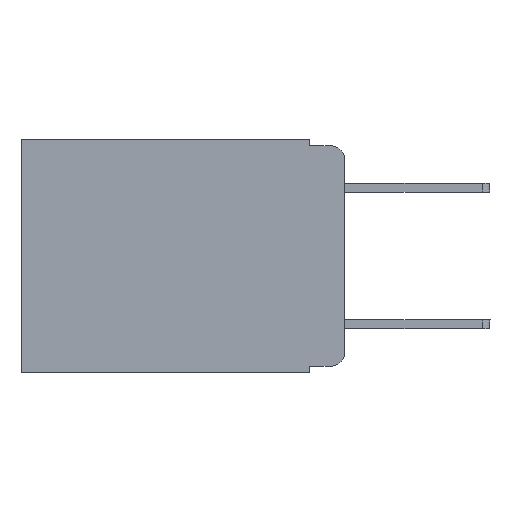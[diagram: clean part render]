
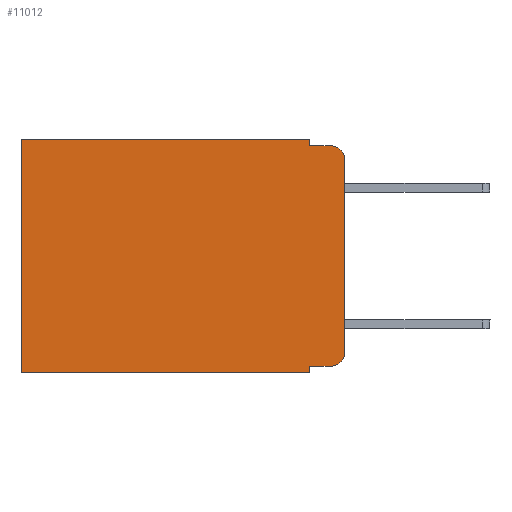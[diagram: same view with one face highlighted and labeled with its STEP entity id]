
A CAD part, left-side view. The second image highlights one B-rep face of the part: STEP entity #11012.
In plain terms, the highlighted planar face has unit normal (-1, 0, 0).
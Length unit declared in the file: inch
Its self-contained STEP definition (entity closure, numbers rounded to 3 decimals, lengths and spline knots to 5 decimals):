
#335 = VERTEX_POINT ( 'NONE', #15757 ) ;
#423 = VERTEX_POINT ( 'NONE', #14371 ) ;
#572 = VECTOR ( 'NONE', #6449, 39.37008 ) ;
#731 = EDGE_CURVE ( 'NONE', #1321, #17641, #1587, .T. ) ;
#1117 = EDGE_CURVE ( 'NONE', #423, #15335, #13544, .T. ) ;
#1249 = CARTESIAN_POINT ( 'NONE',  ( 0.298, 0.473, -0.343 ) ) ;
#1259 = VERTEX_POINT ( 'NONE', #11235 ) ;
#1321 = VERTEX_POINT ( 'NONE', #9311 ) ;
#1359 = LINE ( 'NONE', #6147, #572 ) ;
#1587 = LINE ( 'NONE', #19120, #15562 ) ;
#1827 = CARTESIAN_POINT ( 'NONE',  ( 0.298, 0.02, -0.03 ) ) ;
#2171 = CARTESIAN_POINT ( 'NONE',  ( 0.298, 0., -0.343 ) ) ;
#2373 = DIRECTION ( 'NONE',  ( 0., 1., 0. ) ) ;
#2409 = LINE ( 'NONE', #3792, #13209 ) ;
#2750 = CIRCLE ( 'NONE', #15293, 0.02 ) ;
#2806 = ORIENTED_EDGE ( 'NONE', *, *, #12698, .F. ) ;
#3792 = CARTESIAN_POINT ( 'NONE',  ( 0.298, 0.051, -0.01 ) ) ;
#3807 = CARTESIAN_POINT ( 'NONE',  ( 0.298, 0.02, -0.313 ) ) ;
#3870 = LINE ( 'NONE', #5986, #17325 ) ;
#3873 = EDGE_CURVE ( 'NONE', #10299, #15335, #6056, .T. ) ;
#4924 = VECTOR ( 'NONE', #15930, 39.37008 ) ;
#5332 = CARTESIAN_POINT ( 'NONE',  ( 0.298, 0.051, 0. ) ) ;
#5481 = DIRECTION ( 'NONE',  ( 1., 0., 0. ) ) ;
#5783 = ORIENTED_EDGE ( 'NONE', *, *, #17838, .T. ) ;
#5833 = VERTEX_POINT ( 'NONE', #1249 ) ;
#5986 = CARTESIAN_POINT ( 'NONE',  ( 0.298, 0.473, 0. ) ) ;
#6056 = LINE ( 'NONE', #10724, #9337 ) ;
#6147 = CARTESIAN_POINT ( 'NONE',  ( 0.298, 0.051, 0. ) ) ;
#6407 = EDGE_CURVE ( 'NONE', #7857, #423, #9598, .T. ) ;
#6449 = DIRECTION ( 'NONE',  ( 0., 0., -1. ) ) ;
#6607 = DIRECTION ( 'NONE',  ( 0., 0., -1. ) ) ;
#6977 = CARTESIAN_POINT ( 'NONE',  ( 0.298, 0., -0.313 ) ) ;
#7153 = DIRECTION ( 'NONE',  ( 0., 0., -1. ) ) ;
#7506 = VERTEX_POINT ( 'NONE', #8862 ) ;
#7857 = VERTEX_POINT ( 'NONE', #18734 ) ;
#8014 = CARTESIAN_POINT ( 'NONE',  ( 0.298, 0.051, -0.333 ) ) ;
#8066 = DIRECTION ( 'NONE',  ( 0., 1., 0. ) ) ;
#8364 = EDGE_CURVE ( 'NONE', #1321, #335, #12219, .T. ) ;
#8823 = ORIENTED_EDGE ( 'NONE', *, *, #8364, .F. ) ;
#8862 = CARTESIAN_POINT ( 'NONE',  ( 0.298, 0.051, -0.343 ) ) ;
#8982 = ORIENTED_EDGE ( 'NONE', *, *, #6407, .T. ) ;
#9311 = CARTESIAN_POINT ( 'NONE',  ( 0.298, 0.051, 0. ) ) ;
#9337 = VECTOR ( 'NONE', #13895, 39.37008 ) ;
#9350 = ORIENTED_EDGE ( 'NONE', *, *, #1117, .T. ) ;
#9598 = LINE ( 'NONE', #8014, #10572 ) ;
#10025 = FACE_OUTER_BOUND ( 'NONE', #13487, .T. ) ;
#10299 = VERTEX_POINT ( 'NONE', #19737 ) ;
#10348 = DIRECTION ( 'NONE',  ( 0., 0., -1. ) ) ;
#10572 = VECTOR ( 'NONE', #14577, 39.37008 ) ;
#10634 = ORIENTED_EDGE ( 'NONE', *, *, #3873, .F. ) ;
#10724 = CARTESIAN_POINT ( 'NONE',  ( 0.298, 0., 0. ) ) ;
#11012 = ADVANCED_FACE ( 'NONE', ( #10025 ), #16942, .F. ) ;
#11235 = CARTESIAN_POINT ( 'NONE',  ( 0.298, 0.02, -0.01 ) ) ;
#11397 = AXIS2_PLACEMENT_3D ( 'NONE', #13523, #5481, #10348 ) ;
#11866 = EDGE_CURVE ( 'NONE', #7857, #7506, #1359, .T. ) ;
#12219 = LINE ( 'NONE', #5332, #4924 ) ;
#12698 = EDGE_CURVE ( 'NONE', #7506, #5833, #16829, .T. ) ;
#13128 = VECTOR ( 'NONE', #2373, 39.37008 ) ;
#13209 = VECTOR ( 'NONE', #15245, 39.37008 ) ;
#13445 = ORIENTED_EDGE ( 'NONE', *, *, #15362, .F. ) ;
#13487 = EDGE_LOOP ( 'NONE', ( #10634, #5783, #13445, #8823, #17261, #18360, #2806, #19267, #8982, #9350 ) ) ;
#13523 = CARTESIAN_POINT ( 'NONE',  ( 0.298, 0., 0. ) ) ;
#13544 = CIRCLE ( 'NONE', #16964, 0.02 ) ;
#13895 = DIRECTION ( 'NONE',  ( 0., 0., -1. ) ) ;
#14371 = CARTESIAN_POINT ( 'NONE',  ( 0.298, 0.02, -0.333 ) ) ;
#14577 = DIRECTION ( 'NONE',  ( 0., -1., 0. ) ) ;
#15245 = DIRECTION ( 'NONE',  ( 0., -1., 0. ) ) ;
#15293 = AXIS2_PLACEMENT_3D ( 'NONE', #1827, #19467, #6607 ) ;
#15335 = VERTEX_POINT ( 'NONE', #6977 ) ;
#15362 = EDGE_CURVE ( 'NONE', #335, #1259, #2409, .T. ) ;
#15562 = VECTOR ( 'NONE', #8066, 39.37008 ) ;
#15757 = CARTESIAN_POINT ( 'NONE',  ( 0.298, 0.051, -0.01 ) ) ;
#15930 = DIRECTION ( 'NONE',  ( 0., 0., -1. ) ) ;
#16829 = LINE ( 'NONE', #2171, #13128 ) ;
#16942 = PLANE ( 'NONE',  #11397 ) ;
#16964 = AXIS2_PLACEMENT_3D ( 'NONE', #3807, #20368, #17191 ) ;
#17191 = DIRECTION ( 'NONE',  ( 0., 0., -1. ) ) ;
#17261 = ORIENTED_EDGE ( 'NONE', *, *, #731, .T. ) ;
#17325 = VECTOR ( 'NONE', #7153, 39.37008 ) ;
#17617 = EDGE_CURVE ( 'NONE', #17641, #5833, #3870, .T. ) ;
#17641 = VERTEX_POINT ( 'NONE', #20427 ) ;
#17838 = EDGE_CURVE ( 'NONE', #10299, #1259, #2750, .T. ) ;
#18360 = ORIENTED_EDGE ( 'NONE', *, *, #17617, .T. ) ;
#18734 = CARTESIAN_POINT ( 'NONE',  ( 0.298, 0.051, -0.333 ) ) ;
#19120 = CARTESIAN_POINT ( 'NONE',  ( 0.298, 0., 0. ) ) ;
#19267 = ORIENTED_EDGE ( 'NONE', *, *, #11866, .F. ) ;
#19467 = DIRECTION ( 'NONE',  ( -1., 0., 0. ) ) ;
#19737 = CARTESIAN_POINT ( 'NONE',  ( 0.298, 0., -0.03 ) ) ;
#20368 = DIRECTION ( 'NONE',  ( -1., 0., 0. ) ) ;
#20427 = CARTESIAN_POINT ( 'NONE',  ( 0.298, 0.473, 0. ) ) ;
